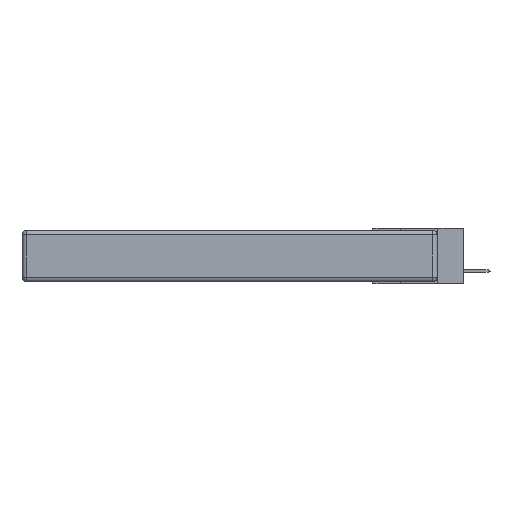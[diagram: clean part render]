
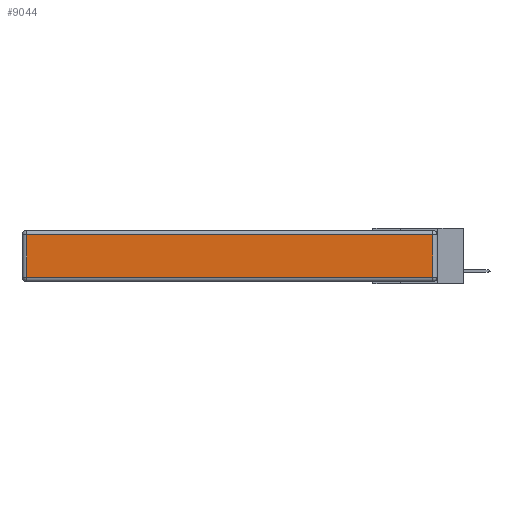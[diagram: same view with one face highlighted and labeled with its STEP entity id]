
A CAD part, left-side view. The second image highlights one B-rep face of the part: STEP entity #9044.
In plain terms, the highlighted planar face has unit normal (-1, 0, 0).
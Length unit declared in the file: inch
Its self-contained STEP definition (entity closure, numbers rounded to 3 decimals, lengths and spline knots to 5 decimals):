
#845 = DIRECTION ( 'NONE',  ( 0., -1., 0. ) ) ;
#1556 = EDGE_CURVE ( 'NONE', #15967, #9005, #8370, .T. ) ;
#1676 = VECTOR ( 'NONE', #845, 39.37008 ) ;
#2288 = FACE_OUTER_BOUND ( 'NONE', #26417, .T. ) ;
#3263 = LINE ( 'NONE', #26166, #1676 ) ;
#6351 = CARTESIAN_POINT ( 'NONE',  ( 0., 2.72, -0.313 ) ) ;
#6428 = ORIENTED_EDGE ( 'NONE', *, *, #13602, .T. ) ;
#6933 = EDGE_CURVE ( 'NONE', #20539, #15967, #3263, .T. ) ;
#7027 = LINE ( 'NONE', #8006, #22533 ) ;
#7226 = CARTESIAN_POINT ( 'NONE',  ( 0., 0.03, -0.313 ) ) ;
#7802 = DIRECTION ( 'NONE',  ( 0., 1., 0. ) ) ;
#8006 = CARTESIAN_POINT ( 'NONE',  ( 0., 2.72, -0.343 ) ) ;
#8370 = LINE ( 'NONE', #17261, #27827 ) ;
#9005 = VERTEX_POINT ( 'NONE', #13049 ) ;
#9044 = ADVANCED_FACE ( 'NONE', ( #2288 ), #29308, .T. ) ;
#10595 = CARTESIAN_POINT ( 'NONE',  ( 0., 2.72, -0.03 ) ) ;
#13049 = CARTESIAN_POINT ( 'NONE',  ( 0., 0.03, -0.03 ) ) ;
#13249 = DIRECTION ( 'NONE',  ( 0., 0., 1. ) ) ;
#13602 = EDGE_CURVE ( 'NONE', #9005, #16760, #19386, .T. ) ;
#14966 = EDGE_CURVE ( 'NONE', #16760, #20539, #7027, .T. ) ;
#15967 = VERTEX_POINT ( 'NONE', #7226 ) ;
#16760 = VERTEX_POINT ( 'NONE', #10595 ) ;
#16881 = DIRECTION ( 'NONE',  ( 0., 0., 1. ) ) ;
#17167 = DIRECTION ( 'NONE',  ( 0., 0., -1. ) ) ;
#17261 = CARTESIAN_POINT ( 'NONE',  ( 0., 0.03, -0.343 ) ) ;
#19386 = LINE ( 'NONE', #21208, #24059 ) ;
#19672 = AXIS2_PLACEMENT_3D ( 'NONE', #26969, #24834, #13249 ) ;
#20089 = ORIENTED_EDGE ( 'NONE', *, *, #14966, .T. ) ;
#20539 = VERTEX_POINT ( 'NONE', #6351 ) ;
#21208 = CARTESIAN_POINT ( 'NONE',  ( 0., 2.75, -0.03 ) ) ;
#22533 = VECTOR ( 'NONE', #17167, 39.37008 ) ;
#24059 = VECTOR ( 'NONE', #7802, 39.37008 ) ;
#24834 = DIRECTION ( 'NONE',  ( -1., 0., 0. ) ) ;
#26166 = CARTESIAN_POINT ( 'NONE',  ( 0., 0., -0.313 ) ) ;
#26417 = EDGE_LOOP ( 'NONE', ( #29826, #26875, #6428, #20089 ) ) ;
#26875 = ORIENTED_EDGE ( 'NONE', *, *, #1556, .T. ) ;
#26969 = CARTESIAN_POINT ( 'NONE',  ( 0., 0., -0.343 ) ) ;
#27827 = VECTOR ( 'NONE', #16881, 39.37008 ) ;
#29308 = PLANE ( 'NONE',  #19672 ) ;
#29826 = ORIENTED_EDGE ( 'NONE', *, *, #6933, .T. ) ;
